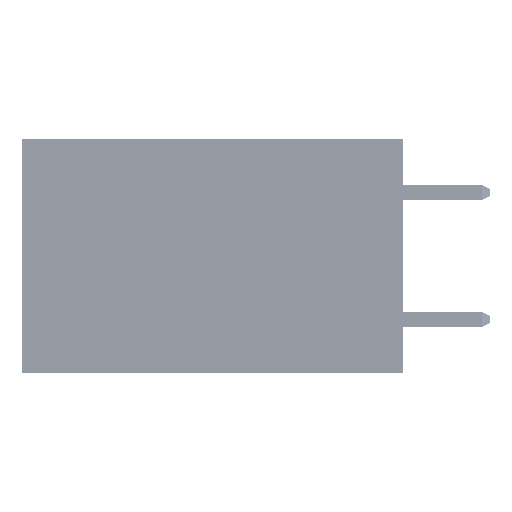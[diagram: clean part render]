
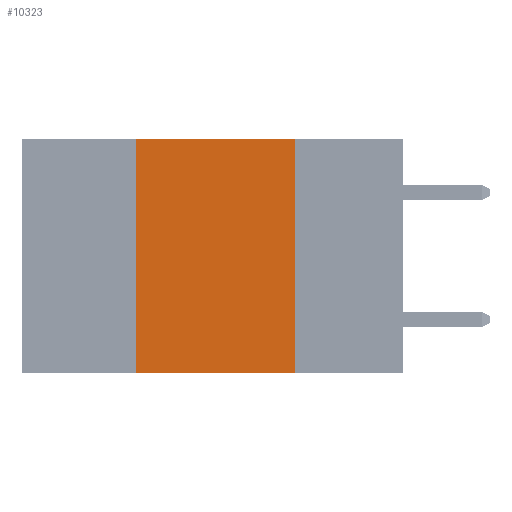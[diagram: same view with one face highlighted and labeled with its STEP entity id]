
A CAD part, left-side view. The second image highlights one B-rep face of the part: STEP entity #10323.
In plain terms, the highlighted planar face has unit normal (-1, 0, 0).
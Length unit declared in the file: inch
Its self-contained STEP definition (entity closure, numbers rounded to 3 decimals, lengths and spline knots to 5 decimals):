
#185 = CARTESIAN_POINT ( 'NONE',  ( 0., 0.42, 0. ) ) ;
#220 = CARTESIAN_POINT ( 'NONE',  ( 0., 0.17, 0. ) ) ;
#920 = DIRECTION ( 'NONE',  ( 0., 0., -1. ) ) ;
#2194 = VECTOR ( 'NONE', #29654, 39.37008 ) ;
#2331 = VECTOR ( 'NONE', #920, 39.37008 ) ;
#2449 = DIRECTION ( 'NONE',  ( 0., 0., 1. ) ) ;
#3839 = CARTESIAN_POINT ( 'NONE',  ( 0., 0.17, -0.37 ) ) ;
#6799 = CARTESIAN_POINT ( 'NONE',  ( 0., 0.17, 0. ) ) ;
#9622 = EDGE_LOOP ( 'NONE', ( #40908, #26806, #17890, #43770 ) ) ;
#10323 = ADVANCED_FACE ( 'NONE', ( #19872 ), #45778, .F. ) ;
#10621 = EDGE_CURVE ( 'NONE', #31693, #33652, #37751, .T. ) ;
#11879 = VECTOR ( 'NONE', #2449, 39.37008 ) ;
#12623 = DIRECTION ( 'NONE',  ( 1., 0., 0. ) ) ;
#17890 = ORIENTED_EDGE ( 'NONE', *, *, #31487, .F. ) ;
#19872 = FACE_OUTER_BOUND ( 'NONE', #9622, .T. ) ;
#20349 = VECTOR ( 'NONE', #30342, 39.37008 ) ;
#20399 = CARTESIAN_POINT ( 'NONE',  ( 0., 0.42, 0. ) ) ;
#22595 = CARTESIAN_POINT ( 'NONE',  ( 0., 0.6, -0.37 ) ) ;
#23307 = LINE ( 'NONE', #22595, #20349 ) ;
#24282 = EDGE_CURVE ( 'NONE', #41020, #31693, #37377, .T. ) ;
#26806 = ORIENTED_EDGE ( 'NONE', *, *, #24282, .F. ) ;
#27167 = LINE ( 'NONE', #20399, #11879 ) ;
#29654 = DIRECTION ( 'NONE',  ( 0., -1., 0. ) ) ;
#30342 = DIRECTION ( 'NONE',  ( 0., -1., 0. ) ) ;
#30921 = AXIS2_PLACEMENT_3D ( 'NONE', #31271, #12623, #46028 ) ;
#31271 = CARTESIAN_POINT ( 'NONE',  ( 0., 0.6, 0. ) ) ;
#31333 = EDGE_CURVE ( 'NONE', #39364, #33652, #23307, .T. ) ;
#31487 = EDGE_CURVE ( 'NONE', #39364, #41020, #27167, .T. ) ;
#31693 = VERTEX_POINT ( 'NONE', #6799 ) ;
#33652 = VERTEX_POINT ( 'NONE', #3839 ) ;
#37207 = CARTESIAN_POINT ( 'NONE',  ( 0., 0.42, -0.37 ) ) ;
#37377 = LINE ( 'NONE', #40287, #2194 ) ;
#37751 = LINE ( 'NONE', #220, #2331 ) ;
#39364 = VERTEX_POINT ( 'NONE', #37207 ) ;
#40287 = CARTESIAN_POINT ( 'NONE',  ( 0., 0.6, 0. ) ) ;
#40908 = ORIENTED_EDGE ( 'NONE', *, *, #10621, .F. ) ;
#41020 = VERTEX_POINT ( 'NONE', #185 ) ;
#43770 = ORIENTED_EDGE ( 'NONE', *, *, #31333, .T. ) ;
#45778 = PLANE ( 'NONE',  #30921 ) ;
#46028 = DIRECTION ( 'NONE',  ( 0., 0., -1. ) ) ;
